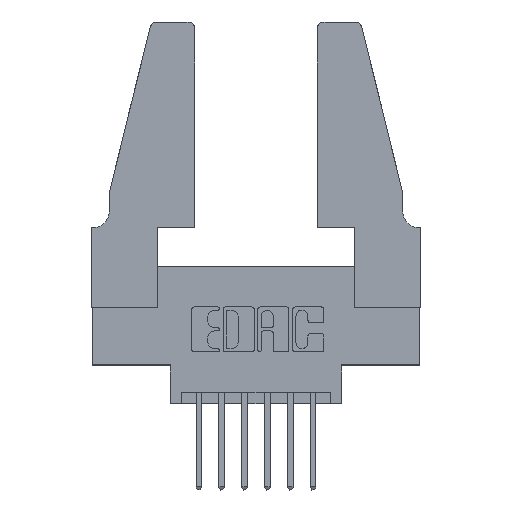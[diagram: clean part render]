
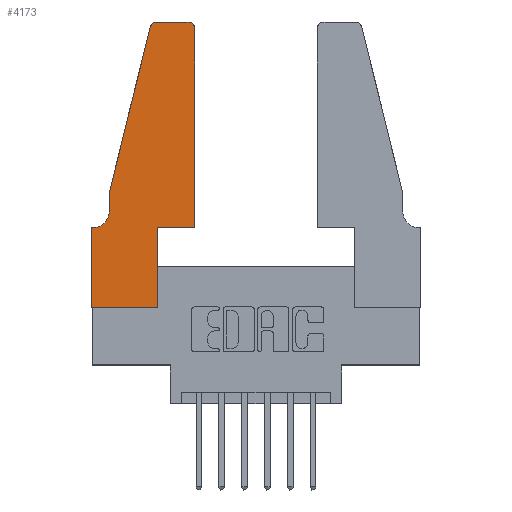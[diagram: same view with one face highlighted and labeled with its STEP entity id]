
A CAD part, top view. The second image highlights one B-rep face of the part: STEP entity #4173.
In plain terms, the highlighted planar face has unit normal (0, 0, 1).
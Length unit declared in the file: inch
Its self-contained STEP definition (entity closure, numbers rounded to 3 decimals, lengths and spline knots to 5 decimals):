
#12 = CARTESIAN_POINT ( 'NONE',  ( 0.4505, 0.35, 0.37 ) ) ;
#143 = CARTESIAN_POINT ( 'NONE',  ( 0., 0., 0.37 ) ) ;
#145 = EDGE_CURVE ( 'NONE', #8797, #2239, #10089, .T. ) ;
#395 = ORIENTED_EDGE ( 'NONE', *, *, #6347, .T. ) ;
#433 = EDGE_CURVE ( 'NONE', #6349, #5328, #5637, .T. ) ;
#542 = CARTESIAN_POINT ( 'NONE',  ( 0.284, 1.22, 0.37 ) ) ;
#599 = CARTESIAN_POINT ( 'NONE',  ( 0., 0.35, 0.37 ) ) ;
#684 = CARTESIAN_POINT ( 'NONE',  ( 0.0755, 0.5, 0.37 ) ) ;
#686 = CARTESIAN_POINT ( 'NONE',  ( 0.0755, 0.5, 0.37 ) ) ;
#923 = CARTESIAN_POINT ( 'NONE',  ( 0.4505, 0.35, 0.37 ) ) ;
#1221 = VERTEX_POINT ( 'NONE', #11571 ) ;
#1344 = AXIS2_PLACEMENT_3D ( 'NONE', #8462, #5723, #2873 ) ;
#1390 = DIRECTION ( 'NONE',  ( 1., 0., 0. ) ) ;
#1435 = PLANE ( 'NONE',  #4706 ) ;
#1451 = DIRECTION ( 'NONE',  ( 1., 0., 0. ) ) ;
#1500 = DIRECTION ( 'NONE',  ( 0., 1., 0. ) ) ;
#1530 = LINE ( 'NONE', #7909, #6991 ) ;
#1565 = VERTEX_POINT ( 'NONE', #5658 ) ;
#1584 = LINE ( 'NONE', #686, #11042 ) ;
#1758 = EDGE_CURVE ( 'NONE', #7329, #4751, #1584, .T. ) ;
#1910 = CARTESIAN_POINT ( 'NONE',  ( 0.0755, 0.42, 0.37 ) ) ;
#2036 = ORIENTED_EDGE ( 'NONE', *, *, #6250, .T. ) ;
#2151 = LINE ( 'NONE', #9468, #6901 ) ;
#2239 = VERTEX_POINT ( 'NONE', #923 ) ;
#2438 = DIRECTION ( 'NONE',  ( 0., 0., 1. ) ) ;
#2798 = CARTESIAN_POINT ( 'NONE',  ( 0., 0., 0.37 ) ) ;
#2873 = DIRECTION ( 'NONE',  ( -1., 0., 0. ) ) ;
#2956 = DIRECTION ( 'NONE',  ( 1., 0., 0. ) ) ;
#3000 = VECTOR ( 'NONE', #3486, 39.37008 ) ;
#3271 = VERTEX_POINT ( 'NONE', #11651 ) ;
#3276 = CARTESIAN_POINT ( 'NONE',  ( 0.0755, 0.35, 0.37 ) ) ;
#3441 = CARTESIAN_POINT ( 'NONE',  ( 0.4205, 1.22, 0.37 ) ) ;
#3486 = DIRECTION ( 'NONE',  ( -1., 0., 0. ) ) ;
#3733 = CARTESIAN_POINT ( 'NONE',  ( 0.4505, 1.22, 0.37 ) ) ;
#3801 = EDGE_CURVE ( 'NONE', #5328, #1221, #1530, .T. ) ;
#4086 = VECTOR ( 'NONE', #11635, 39.37008 ) ;
#4167 = ORIENTED_EDGE ( 'NONE', *, *, #5473, .T. ) ;
#4173 = ADVANCED_FACE ( 'NONE', ( #11029 ), #1435, .T. ) ;
#4237 = ORIENTED_EDGE ( 'NONE', *, *, #8033, .T. ) ;
#4321 = DIRECTION ( 'NONE',  ( 1., 0., 0. ) ) ;
#4325 = CARTESIAN_POINT ( 'NONE',  ( 0.25487, 1.22718, 0.37 ) ) ;
#4399 = VECTOR ( 'NONE', #7454, 39.37008 ) ;
#4706 = AXIS2_PLACEMENT_3D ( 'NONE', #599, #7828, #1390 ) ;
#4751 = VERTEX_POINT ( 'NONE', #1910 ) ;
#4825 = AXIS2_PLACEMENT_3D ( 'NONE', #542, #2438, #1451 ) ;
#4827 = ORIENTED_EDGE ( 'NONE', *, *, #433, .T. ) ;
#4917 = ORIENTED_EDGE ( 'NONE', *, *, #145, .T. ) ;
#5208 = DIRECTION ( 'NONE',  ( 0., 0., 1. ) ) ;
#5315 = CARTESIAN_POINT ( 'NONE',  ( 0.0755, 0.5, 0.37 ) ) ;
#5328 = VERTEX_POINT ( 'NONE', #9609 ) ;
#5429 = LINE ( 'NONE', #3276, #3000 ) ;
#5433 = ORIENTED_EDGE ( 'NONE', *, *, #10559, .T. ) ;
#5473 = EDGE_CURVE ( 'NONE', #3271, #1565, #5429, .T. ) ;
#5485 = DIRECTION ( 'NONE',  ( -0.239, -0.971, 0. ) ) ;
#5544 = CARTESIAN_POINT ( 'NONE',  ( 0.2865, 0., 0.37 ) ) ;
#5637 = CIRCLE ( 'NONE', #11540, 0.03 ) ;
#5658 = CARTESIAN_POINT ( 'NONE',  ( 0., 0.35, 0.37 ) ) ;
#5678 = LINE ( 'NONE', #5315, #7984 ) ;
#5723 = DIRECTION ( 'NONE',  ( 0., 0., -1. ) ) ;
#5994 = CIRCLE ( 'NONE', #1344, 0.07 ) ;
#6017 = DIRECTION ( 'NONE',  ( -1., 0., 0. ) ) ;
#6183 = CIRCLE ( 'NONE', #4825, 0.03 ) ;
#6199 = ORIENTED_EDGE ( 'NONE', *, *, #11592, .T. ) ;
#6250 = EDGE_CURVE ( 'NONE', #4751, #3271, #5994, .T. ) ;
#6275 = ORIENTED_EDGE ( 'NONE', *, *, #1758, .T. ) ;
#6347 = EDGE_CURVE ( 'NONE', #10160, #6876, #7867, .T. ) ;
#6349 = VERTEX_POINT ( 'NONE', #3733 ) ;
#6372 = ORIENTED_EDGE ( 'NONE', *, *, #3801, .T. ) ;
#6800 = ORIENTED_EDGE ( 'NONE', *, *, #10324, .T. ) ;
#6876 = VERTEX_POINT ( 'NONE', #5544 ) ;
#6901 = VECTOR ( 'NONE', #9624, 39.37008 ) ;
#6988 = CARTESIAN_POINT ( 'NONE',  ( 0.2865, 0.35, 0.37 ) ) ;
#6991 = VECTOR ( 'NONE', #6017, 39.37008 ) ;
#7329 = VERTEX_POINT ( 'NONE', #684 ) ;
#7454 = DIRECTION ( 'NONE',  ( 1., 0., 0. ) ) ;
#7828 = DIRECTION ( 'NONE',  ( 0., 0., 1. ) ) ;
#7867 = LINE ( 'NONE', #143, #4399 ) ;
#7909 = CARTESIAN_POINT ( 'NONE',  ( 0.2605, 1.25, 0.37 ) ) ;
#7911 = EDGE_CURVE ( 'NONE', #1565, #10160, #9992, .T. ) ;
#7984 = VECTOR ( 'NONE', #5485, 39.37008 ) ;
#8033 = EDGE_CURVE ( 'NONE', #8431, #7329, #5678, .T. ) ;
#8234 = LINE ( 'NONE', #9702, #8661 ) ;
#8431 = VERTEX_POINT ( 'NONE', #4325 ) ;
#8462 = CARTESIAN_POINT ( 'NONE',  ( 0.0055, 0.42, 0.37 ) ) ;
#8524 = VECTOR ( 'NONE', #2956, 39.37008 ) ;
#8661 = VECTOR ( 'NONE', #1500, 39.37008 ) ;
#8797 = VERTEX_POINT ( 'NONE', #6988 ) ;
#9468 = CARTESIAN_POINT ( 'NONE',  ( 0.4505, 0.35, 0.37 ) ) ;
#9609 = CARTESIAN_POINT ( 'NONE',  ( 0.4205, 1.25, 0.37 ) ) ;
#9624 = DIRECTION ( 'NONE',  ( 0., 1., 0. ) ) ;
#9702 = CARTESIAN_POINT ( 'NONE',  ( 0.2865, 0.35, 0.37 ) ) ;
#9992 = LINE ( 'NONE', #10572, #4086 ) ;
#10089 = LINE ( 'NONE', #12, #8524 ) ;
#10160 = VERTEX_POINT ( 'NONE', #2798 ) ;
#10243 = EDGE_LOOP ( 'NONE', ( #6372, #6199, #4237, #6275, #2036, #4167, #10810, #395, #5433, #4917, #6800, #4827 ) ) ;
#10324 = EDGE_CURVE ( 'NONE', #2239, #6349, #2151, .T. ) ;
#10559 = EDGE_CURVE ( 'NONE', #6876, #8797, #8234, .T. ) ;
#10572 = CARTESIAN_POINT ( 'NONE',  ( 0., 0., 0.37 ) ) ;
#10810 = ORIENTED_EDGE ( 'NONE', *, *, #7911, .T. ) ;
#11029 = FACE_OUTER_BOUND ( 'NONE', #10243, .T. ) ;
#11042 = VECTOR ( 'NONE', #11482, 39.37008 ) ;
#11482 = DIRECTION ( 'NONE',  ( 0., -1., 0. ) ) ;
#11540 = AXIS2_PLACEMENT_3D ( 'NONE', #3441, #5208, #4321 ) ;
#11571 = CARTESIAN_POINT ( 'NONE',  ( 0.284, 1.25, 0.37 ) ) ;
#11592 = EDGE_CURVE ( 'NONE', #1221, #8431, #6183, .T. ) ;
#11635 = DIRECTION ( 'NONE',  ( 0., -1., 0. ) ) ;
#11651 = CARTESIAN_POINT ( 'NONE',  ( 0.0055, 0.35, 0.37 ) ) ;
